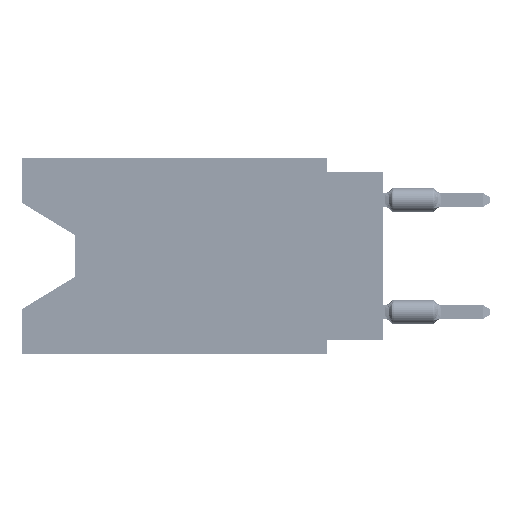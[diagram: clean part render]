
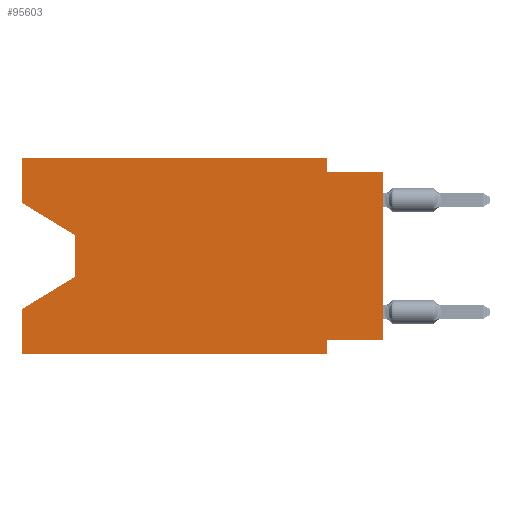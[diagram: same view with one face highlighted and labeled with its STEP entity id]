
A CAD part, left-side view. The second image highlights one B-rep face of the part: STEP entity #95603.
In plain terms, the highlighted planar face has unit normal (-1, 0, 0).
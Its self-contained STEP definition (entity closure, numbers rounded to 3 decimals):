
#419 = EDGE_LOOP ( 'NONE', ( #80042, #12907, #53293, #82879, #8004, #63824, #56019, #36108, #84549, #57278, #75504, #65615 ) ) ;
#789 = LINE ( 'NONE', #40575, #101209 ) ;
#915 = VECTOR ( 'NONE', #36433, 1000. ) ;
#959 = EDGE_CURVE ( 'NONE', #32815, #79014, #72639, .T. ) ;
#1439 = CARTESIAN_POINT ( 'NONE',  ( 0., 0., -8.255 ) ) ;
#2008 = EDGE_CURVE ( 'NONE', #63050, #2378, #789, .T. ) ;
#2378 = VERTEX_POINT ( 'NONE', #54116 ) ;
#4169 = DIRECTION ( 'NONE',  ( 0., -0.855, -0.519 ) ) ;
#6872 = CARTESIAN_POINT ( 'NONE',  ( 0., 13.97, -5.385 ) ) ;
#7680 = DIRECTION ( 'NONE',  ( 1., 0., 0. ) ) ;
#8004 = ORIENTED_EDGE ( 'NONE', *, *, #8807, .T. ) ;
#8716 = DIRECTION ( 'NONE',  ( 0., 0., 1. ) ) ;
#8807 = EDGE_CURVE ( 'NONE', #92570, #84032, #77120, .T. ) ;
#9007 = DIRECTION ( 'NONE',  ( 0., -1., 0. ) ) ;
#9820 = CARTESIAN_POINT ( 'NONE',  ( 0., 16.383, 0. ) ) ;
#9934 = EDGE_CURVE ( 'NONE', #98831, #91868, #90617, .T. ) ;
#11603 = VECTOR ( 'NONE', #99657, 1000. ) ;
#12392 = CARTESIAN_POINT ( 'NONE',  ( 0., 13.97, -5.385 ) ) ;
#12907 = ORIENTED_EDGE ( 'NONE', *, *, #67967, .T. ) ;
#15743 = VECTOR ( 'NONE', #50112, 1000. ) ;
#16646 = CARTESIAN_POINT ( 'NONE',  ( 0., 13.97, -3.505 ) ) ;
#16829 = EDGE_CURVE ( 'NONE', #98831, #71506, #18206, .T. ) ;
#17536 = DIRECTION ( 'NONE',  ( 0., -1., 0. ) ) ;
#18206 = LINE ( 'NONE', #9820, #27390 ) ;
#18379 = EDGE_CURVE ( 'NONE', #19448, #24791, #93843, .T. ) ;
#19448 = VERTEX_POINT ( 'NONE', #12392 ) ;
#19899 = DIRECTION ( 'NONE',  ( 0., 0., 1. ) ) ;
#20388 = EDGE_CURVE ( 'NONE', #81925, #63050, #60001, .T. ) ;
#20861 = CARTESIAN_POINT ( 'NONE',  ( 0., 2.54, 0. ) ) ;
#23714 = CARTESIAN_POINT ( 'NONE',  ( 0., 16.383, -8.89 ) ) ;
#24477 = CARTESIAN_POINT ( 'NONE',  ( 0., 0., -8.255 ) ) ;
#24791 = VERTEX_POINT ( 'NONE', #40954 ) ;
#26687 = VECTOR ( 'NONE', #57193, 1000. ) ;
#27390 = VECTOR ( 'NONE', #41766, 1000. ) ;
#30581 = AXIS2_PLACEMENT_3D ( 'NONE', #102006, #7680, #87821 ) ;
#32815 = VERTEX_POINT ( 'NONE', #1439 ) ;
#35605 = CARTESIAN_POINT ( 'NONE',  ( 0., 16.383, -2.038 ) ) ;
#35959 = CARTESIAN_POINT ( 'NONE',  ( 0., 2.54, -8.89 ) ) ;
#36108 = ORIENTED_EDGE ( 'NONE', *, *, #80990, .T. ) ;
#36433 = DIRECTION ( 'NONE',  ( 0., 0., -1. ) ) ;
#40575 = CARTESIAN_POINT ( 'NONE',  ( 0., 0., -0.635 ) ) ;
#40954 = CARTESIAN_POINT ( 'NONE',  ( 0., 16.383, -6.852 ) ) ;
#40957 = DIRECTION ( 'NONE',  ( 0., 0., -1. ) ) ;
#41766 = DIRECTION ( 'NONE',  ( 0., 0., 1. ) ) ;
#43414 = VECTOR ( 'NONE', #19899, 1000. ) ;
#45295 = VECTOR ( 'NONE', #8716, 1000. ) ;
#45370 = VECTOR ( 'NONE', #4169, 1000. ) ;
#46467 = FACE_OUTER_BOUND ( 'NONE', #419, .T. ) ;
#48539 = LINE ( 'NONE', #80488, #45295 ) ;
#50112 = DIRECTION ( 'NONE',  ( 0., 1., 0. ) ) ;
#53293 = ORIENTED_EDGE ( 'NONE', *, *, #18379, .T. ) ;
#54116 = CARTESIAN_POINT ( 'NONE',  ( 0., 0., -0.635 ) ) ;
#56019 = ORIENTED_EDGE ( 'NONE', *, *, #959, .F. ) ;
#57193 = DIRECTION ( 'NONE',  ( 0., 0., -1. ) ) ;
#57278 = ORIENTED_EDGE ( 'NONE', *, *, #20388, .F. ) ;
#60001 = LINE ( 'NONE', #67327, #915 ) ;
#63050 = VERTEX_POINT ( 'NONE', #71073 ) ;
#63824 = ORIENTED_EDGE ( 'NONE', *, *, #100308, .F. ) ;
#65091 = LINE ( 'NONE', #97046, #26687 ) ;
#65561 = CARTESIAN_POINT ( 'NONE',  ( 0., 16.383, 0. ) ) ;
#65615 = ORIENTED_EDGE ( 'NONE', *, *, #16829, .F. ) ;
#67327 = CARTESIAN_POINT ( 'NONE',  ( 0., 2.54, 0. ) ) ;
#67701 = CARTESIAN_POINT ( 'NONE',  ( 0., 16.383, -8.89 ) ) ;
#67967 = EDGE_CURVE ( 'NONE', #91868, #19448, #65091, .T. ) ;
#69772 = EDGE_CURVE ( 'NONE', #92570, #24791, #76436, .T. ) ;
#70247 = DIRECTION ( 'NONE',  ( 0., 0.855, -0.519 ) ) ;
#71073 = CARTESIAN_POINT ( 'NONE',  ( 0., 2.54, -0.635 ) ) ;
#71506 = VERTEX_POINT ( 'NONE', #79788 ) ;
#72639 = LINE ( 'NONE', #24477, #15743 ) ;
#72889 = LINE ( 'NONE', #102808, #101305 ) ;
#74934 = VECTOR ( 'NONE', #9007, 1000. ) ;
#75504 = ORIENTED_EDGE ( 'NONE', *, *, #91001, .F. ) ;
#76436 = LINE ( 'NONE', #91663, #43414 ) ;
#77017 = CARTESIAN_POINT ( 'NONE',  ( 0., 2.54, -8.255 ) ) ;
#77120 = LINE ( 'NONE', #67701, #11603 ) ;
#79014 = VERTEX_POINT ( 'NONE', #77017 ) ;
#79788 = CARTESIAN_POINT ( 'NONE',  ( 0., 16.383, 0. ) ) ;
#80042 = ORIENTED_EDGE ( 'NONE', *, *, #9934, .T. ) ;
#80488 = CARTESIAN_POINT ( 'NONE',  ( 0., 0., 0. ) ) ;
#80990 = EDGE_CURVE ( 'NONE', #32815, #2378, #48539, .T. ) ;
#81925 = VERTEX_POINT ( 'NONE', #20861 ) ;
#82879 = ORIENTED_EDGE ( 'NONE', *, *, #69772, .F. ) ;
#84032 = VERTEX_POINT ( 'NONE', #35959 ) ;
#84549 = ORIENTED_EDGE ( 'NONE', *, *, #2008, .F. ) ;
#87821 = DIRECTION ( 'NONE',  ( 0., 0., -1. ) ) ;
#90617 = LINE ( 'NONE', #35605, #45370 ) ;
#91001 = EDGE_CURVE ( 'NONE', #71506, #81925, #95981, .T. ) ;
#91663 = CARTESIAN_POINT ( 'NONE',  ( 0., 16.383, 0. ) ) ;
#91868 = VERTEX_POINT ( 'NONE', #16646 ) ;
#92570 = VERTEX_POINT ( 'NONE', #23714 ) ;
#93843 = LINE ( 'NONE', #6872, #97593 ) ;
#95603 = ADVANCED_FACE ( 'NONE', ( #46467 ), #103016, .F. ) ;
#95981 = LINE ( 'NONE', #65561, #74934 ) ;
#97046 = CARTESIAN_POINT ( 'NONE',  ( 0., 13.97, -3.505 ) ) ;
#97593 = VECTOR ( 'NONE', #70247, 1000. ) ;
#97779 = CARTESIAN_POINT ( 'NONE',  ( 0., 16.383, -2.038 ) ) ;
#98831 = VERTEX_POINT ( 'NONE', #97779 ) ;
#99657 = DIRECTION ( 'NONE',  ( 0., -1., 0. ) ) ;
#100308 = EDGE_CURVE ( 'NONE', #79014, #84032, #72889, .T. ) ;
#101209 = VECTOR ( 'NONE', #17536, 1000. ) ;
#101305 = VECTOR ( 'NONE', #40957, 1000. ) ;
#102006 = CARTESIAN_POINT ( 'NONE',  ( 0., 16.383, 0. ) ) ;
#102808 = CARTESIAN_POINT ( 'NONE',  ( 0., 2.54, -8.89 ) ) ;
#103016 = PLANE ( 'NONE',  #30581 ) ;
